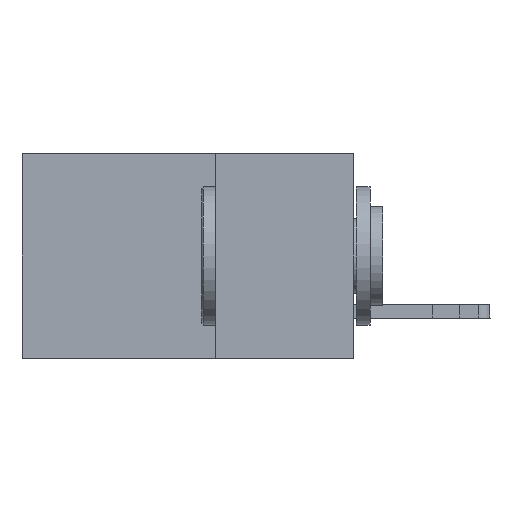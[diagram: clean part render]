
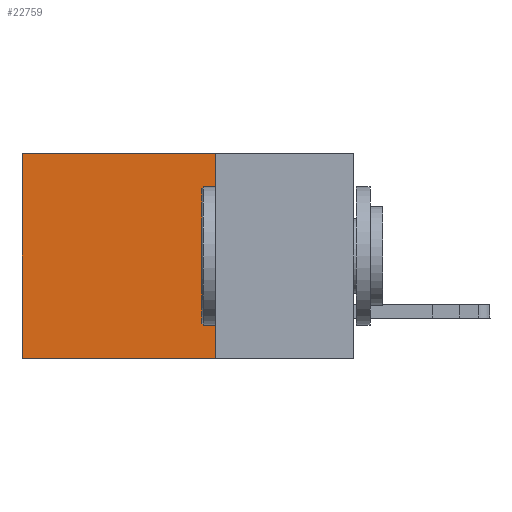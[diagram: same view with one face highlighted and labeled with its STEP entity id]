
A CAD part, left-side view. The second image highlights one B-rep face of the part: STEP entity #22759.
In plain terms, the highlighted planar face has unit normal (-1, 0, 0).
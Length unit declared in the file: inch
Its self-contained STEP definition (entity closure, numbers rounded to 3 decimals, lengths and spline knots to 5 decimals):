
#233 = DIRECTION ( 'NONE',  ( 0., 0., -1. ) ) ;
#1810 = VECTOR ( 'NONE', #233, 39.37008 ) ;
#2331 = CARTESIAN_POINT ( 'NONE',  ( 0.2875, 0.6, -0.37 ) ) ;
#2423 = ORIENTED_EDGE ( 'NONE', *, *, #10050, .T. ) ;
#2508 = VERTEX_POINT ( 'NONE', #21212 ) ;
#3408 = AXIS2_PLACEMENT_3D ( 'NONE', #21939, #19090, #4517 ) ;
#4517 = DIRECTION ( 'NONE',  ( 0., 0., -1. ) ) ;
#5559 = EDGE_CURVE ( 'NONE', #34665, #27481, #12362, .T. ) ;
#7171 = CARTESIAN_POINT ( 'NONE',  ( 0.2875, 0.25, -0.37 ) ) ;
#7746 = VERTEX_POINT ( 'NONE', #26791 ) ;
#8768 = LINE ( 'NONE', #29267, #1810 ) ;
#8775 = CARTESIAN_POINT ( 'NONE',  ( 0.2875, 0.25, 0. ) ) ;
#9852 = DIRECTION ( 'NONE',  ( 0., 1., 0. ) ) ;
#10050 = EDGE_CURVE ( 'NONE', #7746, #2508, #22292, .T. ) ;
#10260 = PLANE ( 'NONE',  #3408 ) ;
#10479 = VECTOR ( 'NONE', #23546, 39.37008 ) ;
#12362 = LINE ( 'NONE', #7171, #19241 ) ;
#13877 = CARTESIAN_POINT ( 'NONE',  ( 0.2875, 0.25, 0. ) ) ;
#14972 = EDGE_CURVE ( 'NONE', #7746, #34665, #28497, .T. ) ;
#18197 = ORIENTED_EDGE ( 'NONE', *, *, #14972, .F. ) ;
#19090 = DIRECTION ( 'NONE',  ( 1., 0., 0. ) ) ;
#19241 = VECTOR ( 'NONE', #9852, 39.37008 ) ;
#19371 = ORIENTED_EDGE ( 'NONE', *, *, #37772, .T. ) ;
#20980 = EDGE_LOOP ( 'NONE', ( #19371, #22039, #18197, #2423 ) ) ;
#21212 = CARTESIAN_POINT ( 'NONE',  ( 0.2875, 0.6, 0. ) ) ;
#21939 = CARTESIAN_POINT ( 'NONE',  ( 0.2875, 0.25, 0. ) ) ;
#22039 = ORIENTED_EDGE ( 'NONE', *, *, #5559, .F. ) ;
#22292 = LINE ( 'NONE', #13877, #26975 ) ;
#22759 = ADVANCED_FACE ( 'NONE', ( #36484 ), #10260, .F. ) ;
#23546 = DIRECTION ( 'NONE',  ( 0., 0., -1. ) ) ;
#26791 = CARTESIAN_POINT ( 'NONE',  ( 0.2875, 0.25, 0. ) ) ;
#26975 = VECTOR ( 'NONE', #27830, 39.37008 ) ;
#27481 = VERTEX_POINT ( 'NONE', #2331 ) ;
#27830 = DIRECTION ( 'NONE',  ( 0., 1., 0. ) ) ;
#28497 = LINE ( 'NONE', #8775, #10479 ) ;
#29267 = CARTESIAN_POINT ( 'NONE',  ( 0.2875, 0.6, 0. ) ) ;
#34665 = VERTEX_POINT ( 'NONE', #37222 ) ;
#36484 = FACE_OUTER_BOUND ( 'NONE', #20980, .T. ) ;
#37222 = CARTESIAN_POINT ( 'NONE',  ( 0.2875, 0.25, -0.37 ) ) ;
#37772 = EDGE_CURVE ( 'NONE', #2508, #27481, #8768, .T. ) ;
